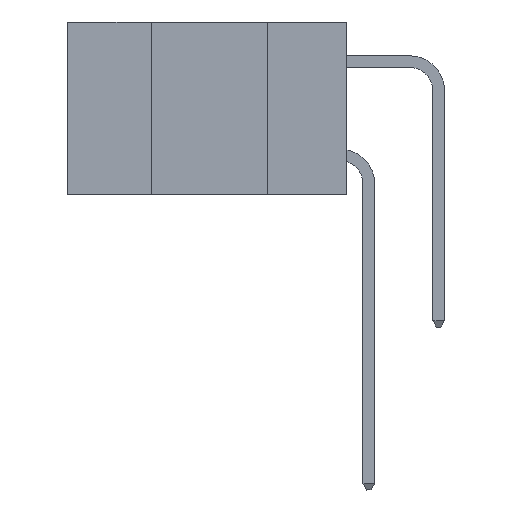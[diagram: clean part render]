
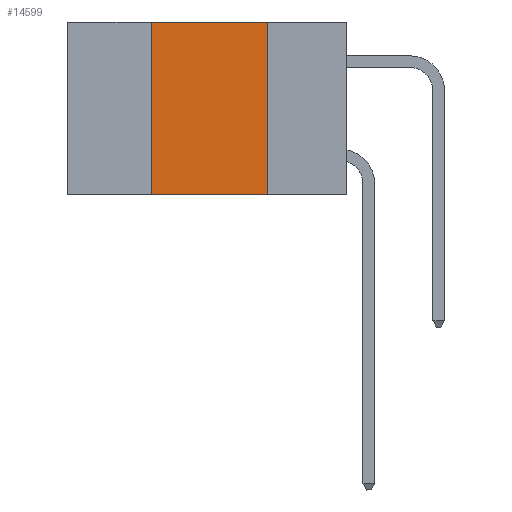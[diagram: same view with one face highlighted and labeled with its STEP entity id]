
A CAD part, left-side view. The second image highlights one B-rep face of the part: STEP entity #14599.
In plain terms, the highlighted planar face has unit normal (-1, 0, 0).
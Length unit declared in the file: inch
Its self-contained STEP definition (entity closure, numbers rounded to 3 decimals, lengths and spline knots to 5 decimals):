
#180 = ORIENTED_EDGE ( 'NONE', *, *, #17057, .F. ) ;
#222 = VERTEX_POINT ( 'NONE', #17496 ) ;
#262 = EDGE_CURVE ( 'NONE', #222, #9204, #3139, .T. ) ;
#311 = EDGE_CURVE ( 'NONE', #222, #10686, #6108, .T. ) ;
#545 = ORIENTED_EDGE ( 'NONE', *, *, #311, .F. ) ;
#980 = VECTOR ( 'NONE', #12129, 39.37008 ) ;
#2074 = VECTOR ( 'NONE', #15658, 39.37008 ) ;
#2378 = DIRECTION ( 'NONE',  ( 0., 0., -1. ) ) ;
#3139 = LINE ( 'NONE', #3495, #19460 ) ;
#3495 = CARTESIAN_POINT ( 'NONE',  ( 0., 0.6, -0.37 ) ) ;
#4450 = ORIENTED_EDGE ( 'NONE', *, *, #10420, .F. ) ;
#4810 = PLANE ( 'NONE',  #9807 ) ;
#6108 = LINE ( 'NONE', #8413, #11570 ) ;
#7688 = CARTESIAN_POINT ( 'NONE',  ( 0., 0.6, 0. ) ) ;
#8413 = CARTESIAN_POINT ( 'NONE',  ( 0., 0.42, 0. ) ) ;
#8563 = CARTESIAN_POINT ( 'NONE',  ( 0., 0.42, 0. ) ) ;
#8796 = DIRECTION ( 'NONE',  ( 1., 0., 0. ) ) ;
#8869 = EDGE_LOOP ( 'NONE', ( #4450, #180, #545, #18542 ) ) ;
#9204 = VERTEX_POINT ( 'NONE', #13189 ) ;
#9807 = AXIS2_PLACEMENT_3D ( 'NONE', #19276, #8796, #2378 ) ;
#10420 = EDGE_CURVE ( 'NONE', #17178, #9204, #10896, .T. ) ;
#10539 = CARTESIAN_POINT ( 'NONE',  ( 0., 0.17, 0. ) ) ;
#10686 = VERTEX_POINT ( 'NONE', #8563 ) ;
#10896 = LINE ( 'NONE', #10539, #980 ) ;
#10999 = LINE ( 'NONE', #7688, #2074 ) ;
#11570 = VECTOR ( 'NONE', #19165, 39.37008 ) ;
#12129 = DIRECTION ( 'NONE',  ( 0., 0., -1. ) ) ;
#13189 = CARTESIAN_POINT ( 'NONE',  ( 0., 0.17, -0.37 ) ) ;
#14599 = ADVANCED_FACE ( 'NONE', ( #14727 ), #4810, .F. ) ;
#14727 = FACE_OUTER_BOUND ( 'NONE', #8869, .T. ) ;
#15658 = DIRECTION ( 'NONE',  ( 0., -1., 0. ) ) ;
#16122 = DIRECTION ( 'NONE',  ( 0., -1., 0. ) ) ;
#17057 = EDGE_CURVE ( 'NONE', #10686, #17178, #10999, .T. ) ;
#17133 = CARTESIAN_POINT ( 'NONE',  ( 0., 0.17, 0. ) ) ;
#17178 = VERTEX_POINT ( 'NONE', #17133 ) ;
#17496 = CARTESIAN_POINT ( 'NONE',  ( 0., 0.42, -0.37 ) ) ;
#18542 = ORIENTED_EDGE ( 'NONE', *, *, #262, .T. ) ;
#19165 = DIRECTION ( 'NONE',  ( 0., 0., 1. ) ) ;
#19276 = CARTESIAN_POINT ( 'NONE',  ( 0., 0.6, 0. ) ) ;
#19460 = VECTOR ( 'NONE', #16122, 39.37008 ) ;
